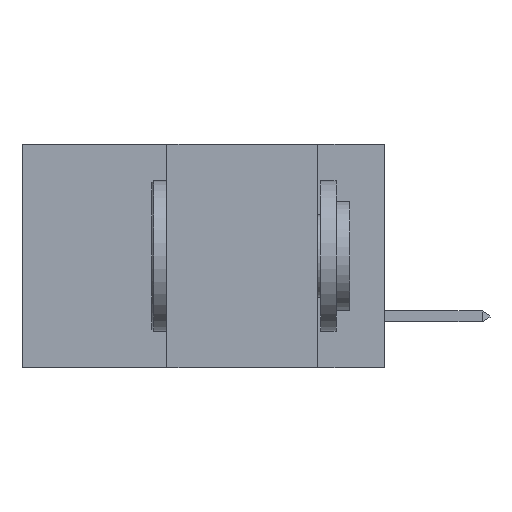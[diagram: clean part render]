
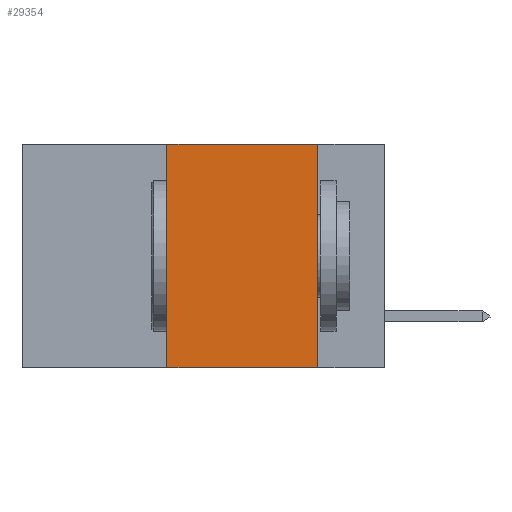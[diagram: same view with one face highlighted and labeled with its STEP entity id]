
A CAD part, left-side view. The second image highlights one B-rep face of the part: STEP entity #29354.
In plain terms, the highlighted planar face has unit normal (-1, 0, 0).
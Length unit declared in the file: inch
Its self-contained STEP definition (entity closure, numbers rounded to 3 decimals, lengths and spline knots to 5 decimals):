
#2807 = DIRECTION ( 'NONE',  ( 0., 0., -1. ) ) ;
#3420 = LINE ( 'NONE', #31472, #23370 ) ;
#3526 = FACE_OUTER_BOUND ( 'NONE', #27283, .T. ) ;
#3841 = DIRECTION ( 'NONE',  ( 0., 0., 1. ) ) ;
#4833 = VERTEX_POINT ( 'NONE', #23993 ) ;
#5603 = CARTESIAN_POINT ( 'NONE',  ( 0., 0.6, 0. ) ) ;
#8164 = ORIENTED_EDGE ( 'NONE', *, *, #21157, .F. ) ;
#8218 = DIRECTION ( 'NONE',  ( 0., 0., -1. ) ) ;
#8638 = AXIS2_PLACEMENT_3D ( 'NONE', #5603, #23807, #8218 ) ;
#8878 = CARTESIAN_POINT ( 'NONE',  ( 0., 0.6, -0.37 ) ) ;
#9405 = VECTOR ( 'NONE', #3841, 39.37008 ) ;
#12445 = VECTOR ( 'NONE', #27132, 39.37008 ) ;
#12627 = VERTEX_POINT ( 'NONE', #27721 ) ;
#13904 = CARTESIAN_POINT ( 'NONE',  ( 0., 0.6, 0. ) ) ;
#15950 = ORIENTED_EDGE ( 'NONE', *, *, #29517, .T. ) ;
#15999 = VERTEX_POINT ( 'NONE', #16354 ) ;
#16342 = LINE ( 'NONE', #27316, #9405 ) ;
#16354 = CARTESIAN_POINT ( 'NONE',  ( 0., 0.36, -0.37 ) ) ;
#16601 = CARTESIAN_POINT ( 'NONE',  ( 0., 0.11, 0. ) ) ;
#17954 = VECTOR ( 'NONE', #29469, 39.37008 ) ;
#21157 = EDGE_CURVE ( 'NONE', #4833, #31719, #26515, .T. ) ;
#21888 = EDGE_CURVE ( 'NONE', #15999, #4833, #16342, .T. ) ;
#23370 = VECTOR ( 'NONE', #2807, 39.37008 ) ;
#23807 = DIRECTION ( 'NONE',  ( 1., 0., 0. ) ) ;
#23993 = CARTESIAN_POINT ( 'NONE',  ( 0., 0.36, 0. ) ) ;
#25522 = LINE ( 'NONE', #8878, #12445 ) ;
#26515 = LINE ( 'NONE', #13904, #17954 ) ;
#27132 = DIRECTION ( 'NONE',  ( 0., -1., 0. ) ) ;
#27283 = EDGE_LOOP ( 'NONE', ( #28521, #8164, #29365, #15950 ) ) ;
#27316 = CARTESIAN_POINT ( 'NONE',  ( 0., 0.36, 0. ) ) ;
#27721 = CARTESIAN_POINT ( 'NONE',  ( 0., 0.11, -0.37 ) ) ;
#28521 = ORIENTED_EDGE ( 'NONE', *, *, #30631, .F. ) ;
#29354 = ADVANCED_FACE ( 'NONE', ( #3526 ), #31548, .F. ) ;
#29365 = ORIENTED_EDGE ( 'NONE', *, *, #21888, .F. ) ;
#29469 = DIRECTION ( 'NONE',  ( 0., -1., 0. ) ) ;
#29517 = EDGE_CURVE ( 'NONE', #15999, #12627, #25522, .T. ) ;
#30631 = EDGE_CURVE ( 'NONE', #31719, #12627, #3420, .T. ) ;
#31472 = CARTESIAN_POINT ( 'NONE',  ( 0., 0.11, 0. ) ) ;
#31548 = PLANE ( 'NONE',  #8638 ) ;
#31719 = VERTEX_POINT ( 'NONE', #16601 ) ;
